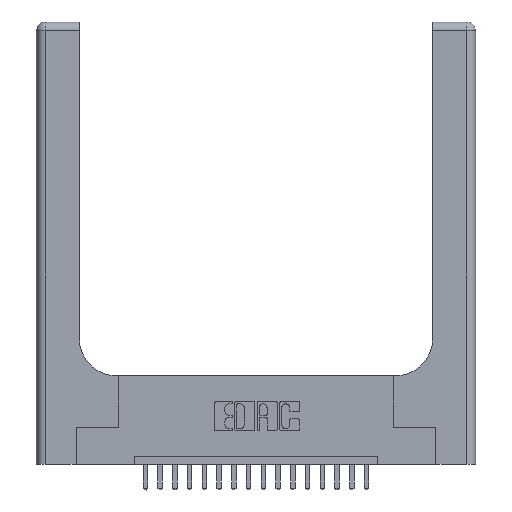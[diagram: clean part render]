
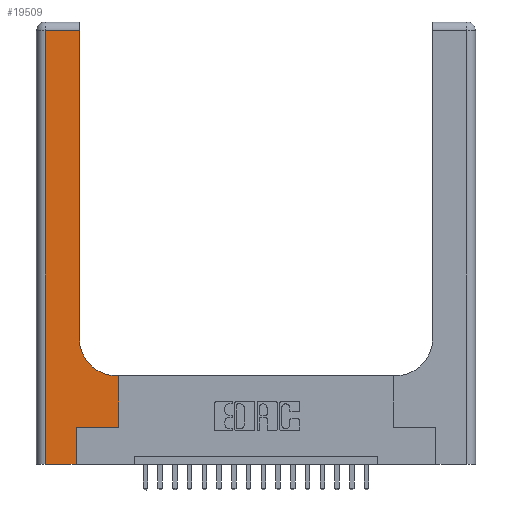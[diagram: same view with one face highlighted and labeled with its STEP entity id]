
A CAD part, top view. The second image highlights one B-rep face of the part: STEP entity #19509.
In plain terms, the highlighted planar face has unit normal (0, 0, 1).
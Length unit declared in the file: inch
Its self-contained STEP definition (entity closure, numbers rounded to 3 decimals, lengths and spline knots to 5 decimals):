
#121 = ORIENTED_EDGE ( 'NONE', *, *, #19679, .T. ) ;
#170 = ORIENTED_EDGE ( 'NONE', *, *, #9130, .T. ) ;
#374 = DIRECTION ( 'NONE',  ( 0., 0., -1. ) ) ;
#582 = DIRECTION ( 'NONE',  ( 1., 0., 0. ) ) ;
#614 = CARTESIAN_POINT ( 'NONE',  ( 0.2915, 3., 0.37 ) ) ;
#772 = CARTESIAN_POINT ( 'NONE',  ( 0.06, 0., 0.37 ) ) ;
#919 = DIRECTION ( 'NONE',  ( -1., 0., 0. ) ) ;
#1037 = DIRECTION ( 'NONE',  ( -1., 0., 0. ) ) ;
#1439 = VECTOR ( 'NONE', #15083, 39.37008 ) ;
#1537 = CARTESIAN_POINT ( 'NONE',  ( 0.269, 0.25, 0.37 ) ) ;
#1691 = LINE ( 'NONE', #614, #1439 ) ;
#1896 = ORIENTED_EDGE ( 'NONE', *, *, #14599, .T. ) ;
#2073 = VERTEX_POINT ( 'NONE', #1537 ) ;
#2494 = DIRECTION ( 'NONE',  ( 0., 1., 0. ) ) ;
#2817 = ORIENTED_EDGE ( 'NONE', *, *, #5976, .T. ) ;
#3316 = ORIENTED_EDGE ( 'NONE', *, *, #12650, .T. ) ;
#4346 = CARTESIAN_POINT ( 'NONE',  ( 0., 2.94, 0.37 ) ) ;
#4511 = CARTESIAN_POINT ( 'NONE',  ( 0., 0., 0.37 ) ) ;
#4920 = VECTOR ( 'NONE', #582, 39.37008 ) ;
#4941 = AXIS2_PLACEMENT_3D ( 'NONE', #10027, #374, #12999 ) ;
#5071 = LINE ( 'NONE', #10370, #17401 ) ;
#5399 = VERTEX_POINT ( 'NONE', #772 ) ;
#5497 = LINE ( 'NONE', #4346, #6023 ) ;
#5684 = LINE ( 'NONE', #17607, #9910 ) ;
#5976 = EDGE_CURVE ( 'NONE', #20086, #18673, #5497, .T. ) ;
#6023 = VECTOR ( 'NONE', #919, 39.37008 ) ;
#6100 = DIRECTION ( 'NONE',  ( 1., 0., 0. ) ) ;
#6393 = DIRECTION ( 'NONE',  ( 0., -1., 0. ) ) ;
#7066 = ORIENTED_EDGE ( 'NONE', *, *, #13064, .T. ) ;
#7320 = ORIENTED_EDGE ( 'NONE', *, *, #17692, .T. ) ;
#8102 = VERTEX_POINT ( 'NONE', #11957 ) ;
#8618 = VECTOR ( 'NONE', #13335, 39.37008 ) ;
#8934 = VECTOR ( 'NONE', #15776, 39.37008 ) ;
#9130 = EDGE_CURVE ( 'NONE', #13570, #20560, #18707, .T. ) ;
#9910 = VECTOR ( 'NONE', #6393, 39.37008 ) ;
#10027 = CARTESIAN_POINT ( 'NONE',  ( 0., 3., 0.37 ) ) ;
#10313 = CARTESIAN_POINT ( 'NONE',  ( 0.269, 0.25, 0.37 ) ) ;
#10370 = CARTESIAN_POINT ( 'NONE',  ( 0.5585, 0.25, 0.37 ) ) ;
#10643 = LINE ( 'NONE', #19665, #8618 ) ;
#11243 = CIRCLE ( 'NONE', #12906, 0.25 ) ;
#11957 = CARTESIAN_POINT ( 'NONE',  ( 0.2915, 0.85, 0.37 ) ) ;
#12546 = DIRECTION ( 'NONE',  ( 0., 0., -1. ) ) ;
#12650 = EDGE_CURVE ( 'NONE', #8102, #20086, #1691, .T. ) ;
#12906 = AXIS2_PLACEMENT_3D ( 'NONE', #20241, #12546, #6100 ) ;
#12999 = DIRECTION ( 'NONE',  ( -1., 0., 0. ) ) ;
#13064 = EDGE_CURVE ( 'NONE', #20560, #8102, #11243, .T. ) ;
#13335 = DIRECTION ( 'NONE',  ( 0., 1., 0. ) ) ;
#13457 = EDGE_CURVE ( 'NONE', #5399, #20328, #18007, .T. ) ;
#13570 = VERTEX_POINT ( 'NONE', #20862 ) ;
#14599 = EDGE_CURVE ( 'NONE', #18673, #5399, #5684, .T. ) ;
#15083 = DIRECTION ( 'NONE',  ( 0., 1., 0. ) ) ;
#15433 = EDGE_CURVE ( 'NONE', #20328, #2073, #10643, .T. ) ;
#15459 = VECTOR ( 'NONE', #1037, 39.37008 ) ;
#15661 = FACE_OUTER_BOUND ( 'NONE', #20312, .T. ) ;
#15776 = DIRECTION ( 'NONE',  ( 1., 0., 0. ) ) ;
#17401 = VECTOR ( 'NONE', #2494, 39.37008 ) ;
#17607 = CARTESIAN_POINT ( 'NONE',  ( 0.06, 3., 0.37 ) ) ;
#17692 = EDGE_CURVE ( 'NONE', #2073, #19666, #20470, .T. ) ;
#18007 = LINE ( 'NONE', #4511, #8934 ) ;
#18063 = PLANE ( 'NONE',  #4941 ) ;
#18106 = CARTESIAN_POINT ( 'NONE',  ( 0.2915, 2.94, 0.37 ) ) ;
#18295 = CARTESIAN_POINT ( 'NONE',  ( 0.06, 2.94, 0.37 ) ) ;
#18673 = VERTEX_POINT ( 'NONE', #18295 ) ;
#18707 = LINE ( 'NONE', #20092, #15459 ) ;
#19509 = ADVANCED_FACE ( 'NONE', ( #15661 ), #18063, .F. ) ;
#19634 = ORIENTED_EDGE ( 'NONE', *, *, #15433, .T. ) ;
#19665 = CARTESIAN_POINT ( 'NONE',  ( 0.269, 0., 0.37 ) ) ;
#19666 = VERTEX_POINT ( 'NONE', #20008 ) ;
#19679 = EDGE_CURVE ( 'NONE', #19666, #13570, #5071, .T. ) ;
#19692 = CARTESIAN_POINT ( 'NONE',  ( 0.5415, 0.6, 0.37 ) ) ;
#19709 = ORIENTED_EDGE ( 'NONE', *, *, #13457, .T. ) ;
#20008 = CARTESIAN_POINT ( 'NONE',  ( 0.5585, 0.25, 0.37 ) ) ;
#20086 = VERTEX_POINT ( 'NONE', #18106 ) ;
#20092 = CARTESIAN_POINT ( 'NONE',  ( 0.2915, 0.6, 0.37 ) ) ;
#20188 = CARTESIAN_POINT ( 'NONE',  ( 0.269, 0., 0.37 ) ) ;
#20241 = CARTESIAN_POINT ( 'NONE',  ( 0.5415, 0.85, 0.37 ) ) ;
#20312 = EDGE_LOOP ( 'NONE', ( #3316, #2817, #1896, #19709, #19634, #7320, #121, #170, #7066 ) ) ;
#20328 = VERTEX_POINT ( 'NONE', #20188 ) ;
#20470 = LINE ( 'NONE', #10313, #4920 ) ;
#20560 = VERTEX_POINT ( 'NONE', #19692 ) ;
#20862 = CARTESIAN_POINT ( 'NONE',  ( 0.5585, 0.6, 0.37 ) ) ;
